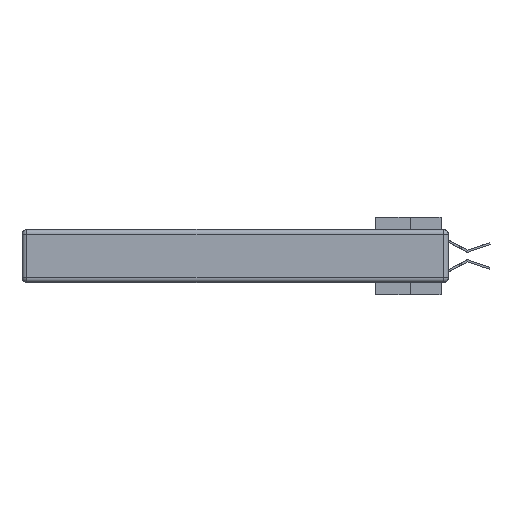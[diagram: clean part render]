
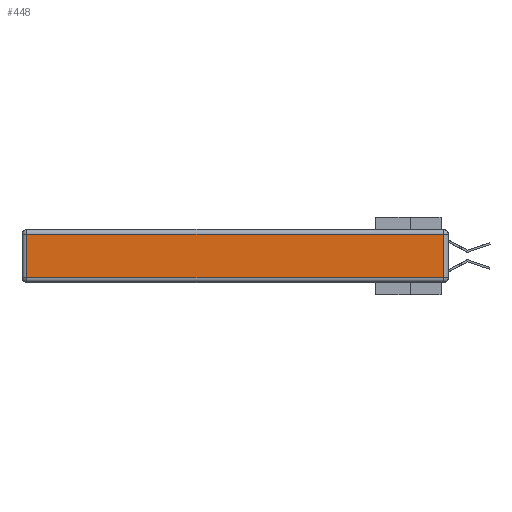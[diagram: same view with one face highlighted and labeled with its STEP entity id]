
A CAD part, left-side view. The second image highlights one B-rep face of the part: STEP entity #448.
In plain terms, the highlighted planar face has unit normal (-1, 0, 0).
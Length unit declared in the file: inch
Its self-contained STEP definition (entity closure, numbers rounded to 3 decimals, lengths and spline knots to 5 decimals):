
#448 = ADVANCED_FACE ( 'NONE', ( #30687 ), #28697, .T. ) ;
#756 = EDGE_CURVE ( 'NONE', #10648, #32573, #4422, .T. ) ;
#2358 = VECTOR ( 'NONE', #29876, 39.37008 ) ;
#4272 = DIRECTION ( 'NONE',  ( 0., -1., 0. ) ) ;
#4422 = LINE ( 'NONE', #19658, #25532 ) ;
#4593 = VERTEX_POINT ( 'NONE', #19269 ) ;
#4773 = ORIENTED_EDGE ( 'NONE', *, *, #17161, .T. ) ;
#6504 = CARTESIAN_POINT ( 'NONE',  ( 0., 2.72, -0.343 ) ) ;
#7670 = ORIENTED_EDGE ( 'NONE', *, *, #24932, .T. ) ;
#8427 = CARTESIAN_POINT ( 'NONE',  ( 0., 0., -0.343 ) ) ;
#10648 = VERTEX_POINT ( 'NONE', #31177 ) ;
#15536 = AXIS2_PLACEMENT_3D ( 'NONE', #8427, #18984, #16216 ) ;
#15640 = CARTESIAN_POINT ( 'NONE',  ( 0., 2.72, -0.313 ) ) ;
#16216 = DIRECTION ( 'NONE',  ( 0., 0., 1. ) ) ;
#16959 = CARTESIAN_POINT ( 'NONE',  ( 0., 0., -0.313 ) ) ;
#17161 = EDGE_CURVE ( 'NONE', #4593, #19009, #31887, .T. ) ;
#18172 = DIRECTION ( 'NONE',  ( 0., 1., 0. ) ) ;
#18655 = LINE ( 'NONE', #16959, #21459 ) ;
#18984 = DIRECTION ( 'NONE',  ( -1., 0., 0. ) ) ;
#19009 = VERTEX_POINT ( 'NONE', #15640 ) ;
#19269 = CARTESIAN_POINT ( 'NONE',  ( 0., 2.72, -0.03 ) ) ;
#19658 = CARTESIAN_POINT ( 'NONE',  ( 0., 0.03, -0.343 ) ) ;
#21008 = LINE ( 'NONE', #30880, #32597 ) ;
#21459 = VECTOR ( 'NONE', #4272, 39.37008 ) ;
#22734 = EDGE_LOOP ( 'NONE', ( #26889, #24992, #7670, #4773 ) ) ;
#24932 = EDGE_CURVE ( 'NONE', #32573, #4593, #21008, .T. ) ;
#24992 = ORIENTED_EDGE ( 'NONE', *, *, #756, .T. ) ;
#25115 = CARTESIAN_POINT ( 'NONE',  ( 0., 0.03, -0.03 ) ) ;
#25532 = VECTOR ( 'NONE', #32701, 39.37008 ) ;
#26889 = ORIENTED_EDGE ( 'NONE', *, *, #30038, .T. ) ;
#28697 = PLANE ( 'NONE',  #15536 ) ;
#29876 = DIRECTION ( 'NONE',  ( 0., 0., -1. ) ) ;
#30038 = EDGE_CURVE ( 'NONE', #19009, #10648, #18655, .T. ) ;
#30687 = FACE_OUTER_BOUND ( 'NONE', #22734, .T. ) ;
#30880 = CARTESIAN_POINT ( 'NONE',  ( 0., 2.75, -0.03 ) ) ;
#31177 = CARTESIAN_POINT ( 'NONE',  ( 0., 0.03, -0.313 ) ) ;
#31887 = LINE ( 'NONE', #6504, #2358 ) ;
#32573 = VERTEX_POINT ( 'NONE', #25115 ) ;
#32597 = VECTOR ( 'NONE', #18172, 39.37008 ) ;
#32701 = DIRECTION ( 'NONE',  ( 0., 0., 1. ) ) ;
